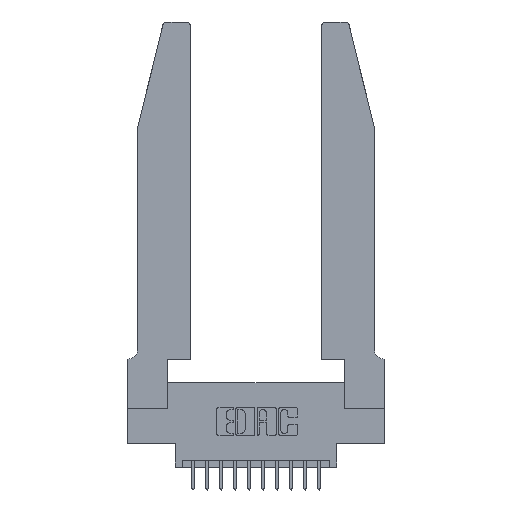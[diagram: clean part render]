
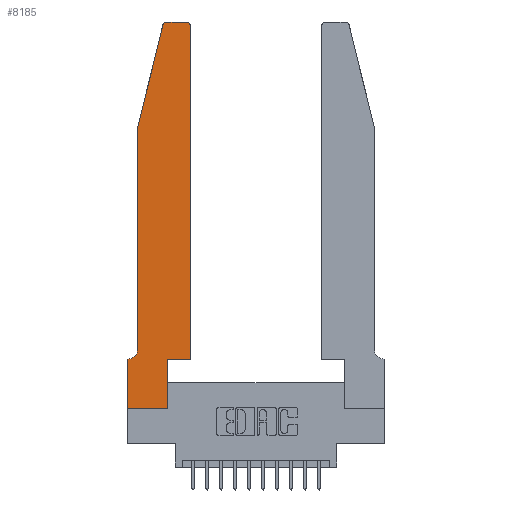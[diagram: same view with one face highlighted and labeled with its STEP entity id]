
A CAD part, top view. The second image highlights one B-rep face of the part: STEP entity #8185.
In plain terms, the highlighted planar face has unit normal (0, 0, 1).
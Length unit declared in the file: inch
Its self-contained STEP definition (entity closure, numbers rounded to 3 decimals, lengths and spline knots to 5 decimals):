
#166 = DIRECTION ( 'NONE',  ( -1., 0., 0. ) ) ;
#472 = CARTESIAN_POINT ( 'NONE',  ( 0.0755, 2., 0.37 ) ) ;
#490 = VERTEX_POINT ( 'NONE', #3051 ) ;
#578 = VERTEX_POINT ( 'NONE', #8658 ) ;
#638 = CARTESIAN_POINT ( 'NONE',  ( 0.284, 2.72, 0.37 ) ) ;
#657 = ORIENTED_EDGE ( 'NONE', *, *, #7010, .T. ) ;
#712 = VECTOR ( 'NONE', #3604, 39.37008 ) ;
#755 = LINE ( 'NONE', #9648, #11898 ) ;
#788 = VERTEX_POINT ( 'NONE', #3712 ) ;
#1081 = DIRECTION ( 'NONE',  ( 0., 0., -1. ) ) ;
#1207 = CARTESIAN_POINT ( 'NONE',  ( 0.0755, 0.42, 0.37 ) ) ;
#1243 = ORIENTED_EDGE ( 'NONE', *, *, #6434, .T. ) ;
#1511 = DIRECTION ( 'NONE',  ( 0., 1., 0. ) ) ;
#1719 = ORIENTED_EDGE ( 'NONE', *, *, #3312, .T. ) ;
#1820 = ORIENTED_EDGE ( 'NONE', *, *, #3581, .T. ) ;
#1922 = DIRECTION ( 'NONE',  ( 0., -1., 0. ) ) ;
#2085 = DIRECTION ( 'NONE',  ( 1., 0., 0. ) ) ;
#2845 = FACE_OUTER_BOUND ( 'NONE', #6147, .T. ) ;
#2903 = VERTEX_POINT ( 'NONE', #11925 ) ;
#3051 = CARTESIAN_POINT ( 'NONE',  ( 0.284, 2.75, 0.37 ) ) ;
#3198 = VECTOR ( 'NONE', #6847, 39.37008 ) ;
#3312 = EDGE_CURVE ( 'NONE', #5637, #14876, #8287, .T. ) ;
#3313 = CARTESIAN_POINT ( 'NONE',  ( 0.4505, 0.35, 0.37 ) ) ;
#3468 = CARTESIAN_POINT ( 'NONE',  ( 0., 0., 0.37 ) ) ;
#3581 = EDGE_CURVE ( 'NONE', #16879, #5038, #8088, .T. ) ;
#3598 = LINE ( 'NONE', #15539, #16987 ) ;
#3604 = DIRECTION ( 'NONE',  ( -0.239, -0.971, 0. ) ) ;
#3712 = CARTESIAN_POINT ( 'NONE',  ( 0., 0.35, 0.37 ) ) ;
#3769 = ORIENTED_EDGE ( 'NONE', *, *, #5277, .T. ) ;
#3855 = EDGE_CURVE ( 'NONE', #578, #490, #4257, .T. ) ;
#3993 = ORIENTED_EDGE ( 'NONE', *, *, #15359, .T. ) ;
#4221 = LINE ( 'NONE', #472, #11620 ) ;
#4231 = AXIS2_PLACEMENT_3D ( 'NONE', #14628, #5690, #14675 ) ;
#4257 = LINE ( 'NONE', #14271, #7878 ) ;
#4290 = DIRECTION ( 'NONE',  ( 0., 0., 1. ) ) ;
#4292 = PLANE ( 'NONE',  #4231 ) ;
#4671 = CARTESIAN_POINT ( 'NONE',  ( 0.2865, 0., 0.37 ) ) ;
#4729 = DIRECTION ( 'NONE',  ( 0., 1., 0. ) ) ;
#4877 = ORIENTED_EDGE ( 'NONE', *, *, #10430, .T. ) ;
#5013 = EDGE_CURVE ( 'NONE', #2903, #12059, #16011, .T. ) ;
#5038 = VERTEX_POINT ( 'NONE', #11296 ) ;
#5277 = EDGE_CURVE ( 'NONE', #15882, #2903, #3598, .T. ) ;
#5448 = CARTESIAN_POINT ( 'NONE',  ( 0., 0., 0.37 ) ) ;
#5608 = DIRECTION ( 'NONE',  ( 1., 0., 0. ) ) ;
#5637 = VERTEX_POINT ( 'NONE', #3468 ) ;
#5690 = DIRECTION ( 'NONE',  ( 0., 0., 1. ) ) ;
#5745 = VECTOR ( 'NONE', #4729, 39.37008 ) ;
#5934 = ORIENTED_EDGE ( 'NONE', *, *, #13338, .T. ) ;
#6147 = EDGE_LOOP ( 'NONE', ( #8438, #5934, #1820, #14067, #1243, #8151, #657, #1719, #4877, #3769, #13882, #3993 ) ) ;
#6434 = EDGE_CURVE ( 'NONE', #9107, #8524, #14419, .T. ) ;
#6617 = DIRECTION ( 'NONE',  ( 1., 0., 0. ) ) ;
#6735 = CARTESIAN_POINT ( 'NONE',  ( 0.2865, 0.35, 0.37 ) ) ;
#6793 = DIRECTION ( 'NONE',  ( 0., -1., 0. ) ) ;
#6847 = DIRECTION ( 'NONE',  ( -1., 0., 0. ) ) ;
#7010 = EDGE_CURVE ( 'NONE', #788, #5637, #9419, .T. ) ;
#7398 = AXIS2_PLACEMENT_3D ( 'NONE', #12135, #4290, #13424 ) ;
#7878 = VECTOR ( 'NONE', #166, 39.37008 ) ;
#7892 = VECTOR ( 'NONE', #5608, 39.37008 ) ;
#7927 = AXIS2_PLACEMENT_3D ( 'NONE', #638, #10152, #2085 ) ;
#8088 = LINE ( 'NONE', #12117, #712 ) ;
#8151 = ORIENTED_EDGE ( 'NONE', *, *, #15282, .T. ) ;
#8185 = ADVANCED_FACE ( 'NONE', ( #2845 ), #4292, .T. ) ;
#8287 = LINE ( 'NONE', #13114, #7892 ) ;
#8438 = ORIENTED_EDGE ( 'NONE', *, *, #3855, .T. ) ;
#8524 = VERTEX_POINT ( 'NONE', #15909 ) ;
#8658 = CARTESIAN_POINT ( 'NONE',  ( 0.4205, 2.75, 0.37 ) ) ;
#8877 = CARTESIAN_POINT ( 'NONE',  ( 0.25487, 2.72718, 0.37 ) ) ;
#9107 = VERTEX_POINT ( 'NONE', #1207 ) ;
#9260 = CARTESIAN_POINT ( 'NONE',  ( 0.0055, 0.42, 0.37 ) ) ;
#9419 = LINE ( 'NONE', #5448, #15804 ) ;
#9458 = CARTESIAN_POINT ( 'NONE',  ( 0.0755, 0.35, 0.37 ) ) ;
#9648 = CARTESIAN_POINT ( 'NONE',  ( 0.2865, 0.35, 0.37 ) ) ;
#10152 = DIRECTION ( 'NONE',  ( 0., 0., 1. ) ) ;
#10348 = CIRCLE ( 'NONE', #7927, 0.03 ) ;
#10430 = EDGE_CURVE ( 'NONE', #14876, #15882, #755, .T. ) ;
#10536 = DIRECTION ( 'NONE',  ( -1., 0., 0. ) ) ;
#11296 = CARTESIAN_POINT ( 'NONE',  ( 0.0755, 2., 0.37 ) ) ;
#11620 = VECTOR ( 'NONE', #1922, 39.37008 ) ;
#11898 = VECTOR ( 'NONE', #1511, 39.37008 ) ;
#11925 = CARTESIAN_POINT ( 'NONE',  ( 0.4505, 0.35, 0.37 ) ) ;
#12059 = VERTEX_POINT ( 'NONE', #12453 ) ;
#12117 = CARTESIAN_POINT ( 'NONE',  ( 0.0755, 2., 0.37 ) ) ;
#12135 = CARTESIAN_POINT ( 'NONE',  ( 0.4205, 2.72, 0.37 ) ) ;
#12452 = CIRCLE ( 'NONE', #7398, 0.03 ) ;
#12453 = CARTESIAN_POINT ( 'NONE',  ( 0.4505, 2.72, 0.37 ) ) ;
#13114 = CARTESIAN_POINT ( 'NONE',  ( 0., 0., 0.37 ) ) ;
#13191 = AXIS2_PLACEMENT_3D ( 'NONE', #9260, #1081, #10536 ) ;
#13338 = EDGE_CURVE ( 'NONE', #490, #16879, #10348, .T. ) ;
#13424 = DIRECTION ( 'NONE',  ( 1., 0., 0. ) ) ;
#13882 = ORIENTED_EDGE ( 'NONE', *, *, #5013, .T. ) ;
#14067 = ORIENTED_EDGE ( 'NONE', *, *, #16794, .T. ) ;
#14271 = CARTESIAN_POINT ( 'NONE',  ( 0.2605, 2.75, 0.37 ) ) ;
#14419 = CIRCLE ( 'NONE', #13191, 0.07 ) ;
#14628 = CARTESIAN_POINT ( 'NONE',  ( 0., 0.35, 0.37 ) ) ;
#14675 = DIRECTION ( 'NONE',  ( 1., 0., 0. ) ) ;
#14876 = VERTEX_POINT ( 'NONE', #4671 ) ;
#15282 = EDGE_CURVE ( 'NONE', #8524, #788, #16637, .T. ) ;
#15359 = EDGE_CURVE ( 'NONE', #12059, #578, #12452, .T. ) ;
#15539 = CARTESIAN_POINT ( 'NONE',  ( 0.4505, 0.35, 0.37 ) ) ;
#15804 = VECTOR ( 'NONE', #6793, 39.37008 ) ;
#15882 = VERTEX_POINT ( 'NONE', #6735 ) ;
#15909 = CARTESIAN_POINT ( 'NONE',  ( 0.0055, 0.35, 0.37 ) ) ;
#16011 = LINE ( 'NONE', #3313, #5745 ) ;
#16637 = LINE ( 'NONE', #9458, #3198 ) ;
#16794 = EDGE_CURVE ( 'NONE', #5038, #9107, #4221, .T. ) ;
#16879 = VERTEX_POINT ( 'NONE', #8877 ) ;
#16987 = VECTOR ( 'NONE', #6617, 39.37008 ) ;
